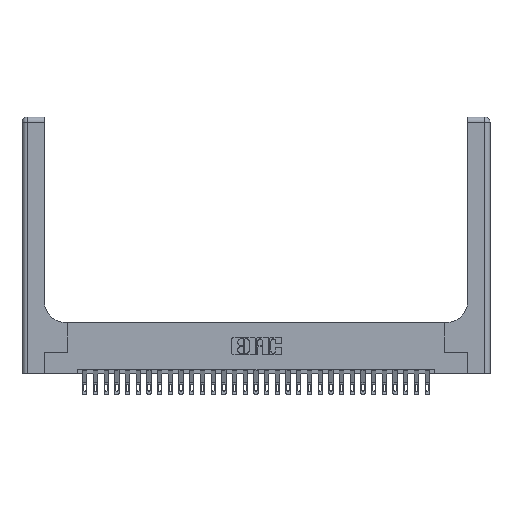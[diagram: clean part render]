
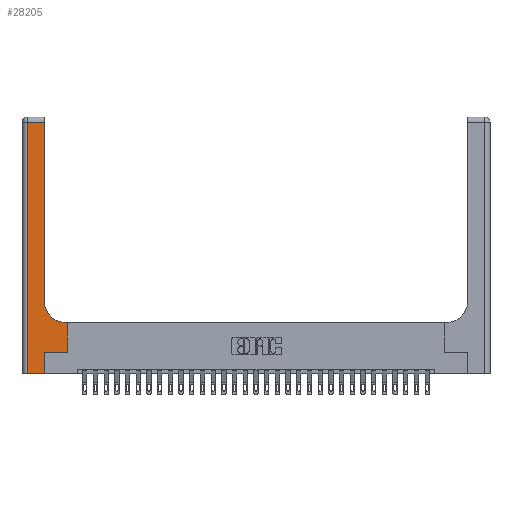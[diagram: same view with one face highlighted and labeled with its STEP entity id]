
A CAD part, top view. The second image highlights one B-rep face of the part: STEP entity #28205.
In plain terms, the highlighted planar face has unit normal (0, 0, 1).
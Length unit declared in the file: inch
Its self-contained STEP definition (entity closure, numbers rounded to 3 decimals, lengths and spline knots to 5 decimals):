
#277 = DIRECTION ( 'NONE',  ( 1., 0., 0. ) ) ;
#737 = DIRECTION ( 'NONE',  ( 0., 1., 0. ) ) ;
#796 = ORIENTED_EDGE ( 'NONE', *, *, #16432, .T. ) ;
#1052 = VERTEX_POINT ( 'NONE', #22227 ) ;
#1474 = VERTEX_POINT ( 'NONE', #7112 ) ;
#1947 = DIRECTION ( 'NONE',  ( -1., 0., 0. ) ) ;
#2802 = AXIS2_PLACEMENT_3D ( 'NONE', #12984, #21840, #1947 ) ;
#3267 = VERTEX_POINT ( 'NONE', #6302 ) ;
#3497 = CARTESIAN_POINT ( 'NONE',  ( 0.06, 3., 0.37 ) ) ;
#3822 = DIRECTION ( 'NONE',  ( -1., 0., 0. ) ) ;
#4476 = ORIENTED_EDGE ( 'NONE', *, *, #26101, .T. ) ;
#4625 = ORIENTED_EDGE ( 'NONE', *, *, #26333, .T. ) ;
#4764 = CARTESIAN_POINT ( 'NONE',  ( 0., 0., 0.37 ) ) ;
#5043 = ORIENTED_EDGE ( 'NONE', *, *, #25906, .T. ) ;
#5049 = AXIS2_PLACEMENT_3D ( 'NONE', #9063, #17930, #6900 ) ;
#5988 = VECTOR ( 'NONE', #7299, 39.37008 ) ;
#6302 = CARTESIAN_POINT ( 'NONE',  ( 0.528, 0.6, 0.37 ) ) ;
#6900 = DIRECTION ( 'NONE',  ( 1., 0., 0. ) ) ;
#6953 = LINE ( 'NONE', #4764, #14287 ) ;
#7112 = CARTESIAN_POINT ( 'NONE',  ( 0.265, 0., 0.37 ) ) ;
#7129 = ORIENTED_EDGE ( 'NONE', *, *, #20407, .T. ) ;
#7299 = DIRECTION ( 'NONE',  ( 0., 1., 0. ) ) ;
#8355 = FACE_OUTER_BOUND ( 'NONE', #24616, .T. ) ;
#8685 = DIRECTION ( 'NONE',  ( 1., 0., 0. ) ) ;
#9063 = CARTESIAN_POINT ( 'NONE',  ( 0.51, 0.85, 0.37 ) ) ;
#9483 = VECTOR ( 'NONE', #23239, 39.37008 ) ;
#9617 = LINE ( 'NONE', #27041, #5988 ) ;
#10891 = CARTESIAN_POINT ( 'NONE',  ( 0.265, 0.25, 0.37 ) ) ;
#11425 = LINE ( 'NONE', #27104, #17462 ) ;
#11452 = VECTOR ( 'NONE', #277, 39.37008 ) ;
#11514 = VERTEX_POINT ( 'NONE', #19757 ) ;
#11704 = ORIENTED_EDGE ( 'NONE', *, *, #11975, .T. ) ;
#11775 = VERTEX_POINT ( 'NONE', #13952 ) ;
#11975 = EDGE_CURVE ( 'NONE', #11514, #21269, #23963, .T. ) ;
#12199 = VERTEX_POINT ( 'NONE', #18427 ) ;
#12921 = CIRCLE ( 'NONE', #5049, 0.25 ) ;
#12984 = CARTESIAN_POINT ( 'NONE',  ( 0., 3., 0.37 ) ) ;
#13012 = VERTEX_POINT ( 'NONE', #20079 ) ;
#13124 = EDGE_CURVE ( 'NONE', #13012, #12199, #16731, .T. ) ;
#13952 = CARTESIAN_POINT ( 'NONE',  ( 0.51, 0.6, 0.37 ) ) ;
#14287 = VECTOR ( 'NONE', #8685, 39.37008 ) ;
#14598 = VERTEX_POINT ( 'NONE', #19648 ) ;
#15201 = ORIENTED_EDGE ( 'NONE', *, *, #18493, .T. ) ;
#16428 = CARTESIAN_POINT ( 'NONE',  ( 0.26, 0.6, 0.37 ) ) ;
#16432 = EDGE_CURVE ( 'NONE', #3267, #11775, #25850, .T. ) ;
#16731 = LINE ( 'NONE', #25001, #19110 ) ;
#17198 = ORIENTED_EDGE ( 'NONE', *, *, #22325, .T. ) ;
#17462 = VECTOR ( 'NONE', #22738, 39.37008 ) ;
#17930 = DIRECTION ( 'NONE',  ( 0., 0., -1. ) ) ;
#18427 = CARTESIAN_POINT ( 'NONE',  ( 0.26, 2.94, 0.37 ) ) ;
#18493 = EDGE_CURVE ( 'NONE', #14598, #3267, #11425, .T. ) ;
#18637 = ORIENTED_EDGE ( 'NONE', *, *, #13124, .T. ) ;
#19110 = VECTOR ( 'NONE', #737, 39.37008 ) ;
#19648 = CARTESIAN_POINT ( 'NONE',  ( 0.528, 0.25, 0.37 ) ) ;
#19757 = CARTESIAN_POINT ( 'NONE',  ( 0.06, 2.94, 0.37 ) ) ;
#20079 = CARTESIAN_POINT ( 'NONE',  ( 0.26, 0.85, 0.37 ) ) ;
#20407 = EDGE_CURVE ( 'NONE', #1052, #14598, #26722, .T. ) ;
#21115 = LINE ( 'NONE', #23288, #26854 ) ;
#21269 = VERTEX_POINT ( 'NONE', #27707 ) ;
#21840 = DIRECTION ( 'NONE',  ( 0., 0., -1. ) ) ;
#22227 = CARTESIAN_POINT ( 'NONE',  ( 0.265, 0.25, 0.37 ) ) ;
#22325 = EDGE_CURVE ( 'NONE', #21269, #1474, #6953, .T. ) ;
#22738 = DIRECTION ( 'NONE',  ( 0., 1., 0. ) ) ;
#23239 = DIRECTION ( 'NONE',  ( -1., 0., 0. ) ) ;
#23288 = CARTESIAN_POINT ( 'NONE',  ( 0., 2.94, 0.37 ) ) ;
#23963 = LINE ( 'NONE', #3497, #27482 ) ;
#24040 = PLANE ( 'NONE',  #2802 ) ;
#24616 = EDGE_LOOP ( 'NONE', ( #18637, #4476, #11704, #17198, #4625, #7129, #15201, #796, #5043 ) ) ;
#25001 = CARTESIAN_POINT ( 'NONE',  ( 0.26, 3., 0.37 ) ) ;
#25711 = DIRECTION ( 'NONE',  ( 0., -1., 0. ) ) ;
#25850 = LINE ( 'NONE', #16428, #9483 ) ;
#25906 = EDGE_CURVE ( 'NONE', #11775, #13012, #12921, .T. ) ;
#26101 = EDGE_CURVE ( 'NONE', #12199, #11514, #21115, .T. ) ;
#26333 = EDGE_CURVE ( 'NONE', #1474, #1052, #9617, .T. ) ;
#26722 = LINE ( 'NONE', #10891, #11452 ) ;
#26854 = VECTOR ( 'NONE', #3822, 39.37008 ) ;
#27041 = CARTESIAN_POINT ( 'NONE',  ( 0.265, 0., 0.37 ) ) ;
#27104 = CARTESIAN_POINT ( 'NONE',  ( 0.528, 0.25, 0.37 ) ) ;
#27482 = VECTOR ( 'NONE', #25711, 39.37008 ) ;
#27707 = CARTESIAN_POINT ( 'NONE',  ( 0.06, 0., 0.37 ) ) ;
#28205 = ADVANCED_FACE ( 'NONE', ( #8355 ), #24040, .F. ) ;
